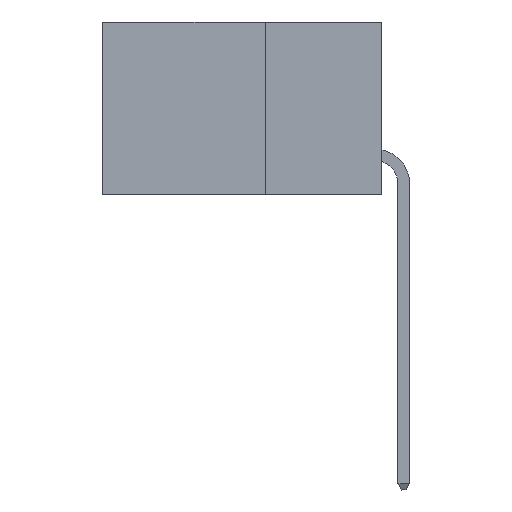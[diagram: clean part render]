
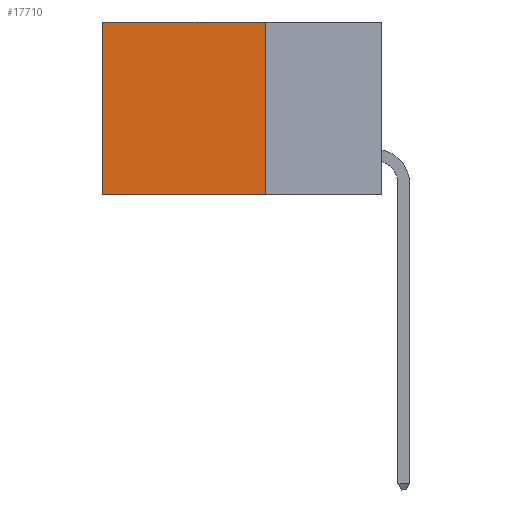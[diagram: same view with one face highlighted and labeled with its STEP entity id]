
A CAD part, left-side view. The second image highlights one B-rep face of the part: STEP entity #17710.
In plain terms, the highlighted planar face has unit normal (-1, 0, 0).
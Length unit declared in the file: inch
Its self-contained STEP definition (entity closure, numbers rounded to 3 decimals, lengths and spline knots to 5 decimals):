
#157 = DIRECTION ( 'NONE',  ( 0., 1., 0. ) ) ;
#305 = VERTEX_POINT ( 'NONE', #17902 ) ;
#401 = VECTOR ( 'NONE', #157, 39.37008 ) ;
#976 = LINE ( 'NONE', #1632, #22767 ) ;
#1632 = CARTESIAN_POINT ( 'NONE',  ( 0.2875, 0.6, 0. ) ) ;
#2434 = EDGE_CURVE ( 'NONE', #22606, #305, #6003, .T. ) ;
#2507 = EDGE_LOOP ( 'NONE', ( #19025, #22134, #14158, #20249 ) ) ;
#6003 = LINE ( 'NONE', #12708, #401 ) ;
#6007 = VERTEX_POINT ( 'NONE', #20919 ) ;
#9233 = LINE ( 'NONE', #22454, #24795 ) ;
#9273 = DIRECTION ( 'NONE',  ( 1., 0., 0. ) ) ;
#9751 = DIRECTION ( 'NONE',  ( 0., 1., 0. ) ) ;
#10558 = LINE ( 'NONE', #10920, #21207 ) ;
#10920 = CARTESIAN_POINT ( 'NONE',  ( 0.2875, 0.25, 0. ) ) ;
#11900 = EDGE_CURVE ( 'NONE', #6007, #23739, #9233, .T. ) ;
#12708 = CARTESIAN_POINT ( 'NONE',  ( 0.2875, 0.25, -0.37 ) ) ;
#13712 = CARTESIAN_POINT ( 'NONE',  ( 0.2875, 0.6, 0. ) ) ;
#14158 = ORIENTED_EDGE ( 'NONE', *, *, #24464, .F. ) ;
#16302 = DIRECTION ( 'NONE',  ( 0., 0., -1. ) ) ;
#16352 = AXIS2_PLACEMENT_3D ( 'NONE', #21965, #9273, #24078 ) ;
#17710 = ADVANCED_FACE ( 'NONE', ( #25450 ), #19813, .F. ) ;
#17902 = CARTESIAN_POINT ( 'NONE',  ( 0.2875, 0.6, -0.37 ) ) ;
#18607 = CARTESIAN_POINT ( 'NONE',  ( 0.2875, 0.25, -0.37 ) ) ;
#18698 = EDGE_CURVE ( 'NONE', #23739, #305, #976, .T. ) ;
#19025 = ORIENTED_EDGE ( 'NONE', *, *, #18698, .T. ) ;
#19813 = PLANE ( 'NONE',  #16352 ) ;
#20249 = ORIENTED_EDGE ( 'NONE', *, *, #11900, .T. ) ;
#20905 = DIRECTION ( 'NONE',  ( 0., 0., -1. ) ) ;
#20919 = CARTESIAN_POINT ( 'NONE',  ( 0.2875, 0.25, 0. ) ) ;
#21207 = VECTOR ( 'NONE', #20905, 39.37008 ) ;
#21965 = CARTESIAN_POINT ( 'NONE',  ( 0.2875, 0.25, 0. ) ) ;
#22134 = ORIENTED_EDGE ( 'NONE', *, *, #2434, .F. ) ;
#22454 = CARTESIAN_POINT ( 'NONE',  ( 0.2875, 0.25, 0. ) ) ;
#22606 = VERTEX_POINT ( 'NONE', #18607 ) ;
#22767 = VECTOR ( 'NONE', #16302, 39.37008 ) ;
#23739 = VERTEX_POINT ( 'NONE', #13712 ) ;
#24078 = DIRECTION ( 'NONE',  ( 0., 0., -1. ) ) ;
#24464 = EDGE_CURVE ( 'NONE', #6007, #22606, #10558, .T. ) ;
#24795 = VECTOR ( 'NONE', #9751, 39.37008 ) ;
#25450 = FACE_OUTER_BOUND ( 'NONE', #2507, .T. ) ;
